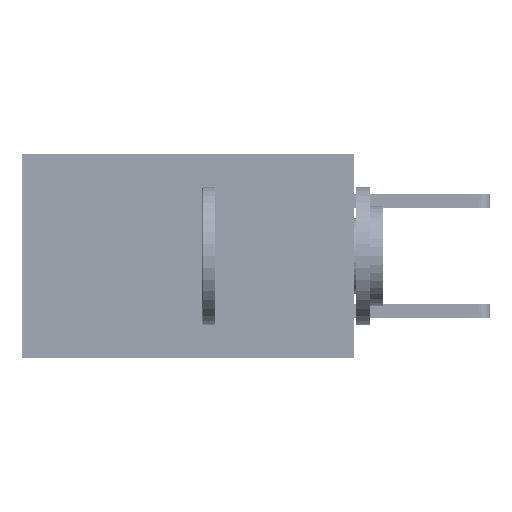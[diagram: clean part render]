
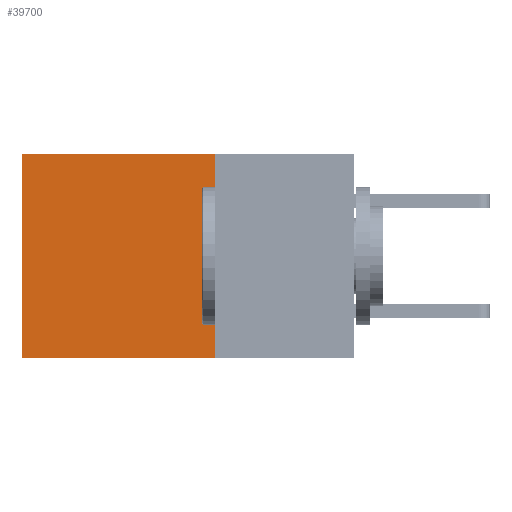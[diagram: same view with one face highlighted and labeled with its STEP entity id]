
A CAD part, left-side view. The second image highlights one B-rep face of the part: STEP entity #39700.
In plain terms, the highlighted planar face has unit normal (-1, 0, 0).
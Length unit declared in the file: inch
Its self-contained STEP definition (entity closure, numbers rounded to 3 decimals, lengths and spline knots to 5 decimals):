
#5642 = EDGE_LOOP ( 'NONE', ( #17971, #10658, #11846, #21129 ) ) ;
#6318 = CARTESIAN_POINT ( 'NONE',  ( 0.2875, 0.25, 0. ) ) ;
#7401 = CARTESIAN_POINT ( 'NONE',  ( 0.2875, 0.6, -0.37 ) ) ;
#7783 = FACE_OUTER_BOUND ( 'NONE', #5642, .T. ) ;
#10658 = ORIENTED_EDGE ( 'NONE', *, *, #20446, .F. ) ;
#11663 = VERTEX_POINT ( 'NONE', #6318 ) ;
#11846 = ORIENTED_EDGE ( 'NONE', *, *, #44434, .F. ) ;
#13267 = LINE ( 'NONE', #27646, #29288 ) ;
#13630 = VERTEX_POINT ( 'NONE', #45906 ) ;
#15787 = CARTESIAN_POINT ( 'NONE',  ( 0.2875, 0.25, 0. ) ) ;
#15796 = LINE ( 'NONE', #33018, #42205 ) ;
#16317 = VECTOR ( 'NONE', #34001, 39.37008 ) ;
#17438 = VERTEX_POINT ( 'NONE', #7401 ) ;
#17971 = ORIENTED_EDGE ( 'NONE', *, *, #22634, .T. ) ;
#20446 = EDGE_CURVE ( 'NONE', #41183, #17438, #13267, .T. ) ;
#21129 = ORIENTED_EDGE ( 'NONE', *, *, #32386, .T. ) ;
#22634 = EDGE_CURVE ( 'NONE', #13630, #17438, #15796, .T. ) ;
#23850 = DIRECTION ( 'NONE',  ( 0., 0., -1. ) ) ;
#24641 = AXIS2_PLACEMENT_3D ( 'NONE', #15787, #40311, #30155 ) ;
#27170 = LINE ( 'NONE', #27402, #16317 ) ;
#27402 = CARTESIAN_POINT ( 'NONE',  ( 0.2875, 0.25, 0. ) ) ;
#27646 = CARTESIAN_POINT ( 'NONE',  ( 0.2875, 0.25, -0.37 ) ) ;
#29288 = VECTOR ( 'NONE', #42021, 39.37008 ) ;
#30155 = DIRECTION ( 'NONE',  ( 0., 0., -1. ) ) ;
#30162 = DIRECTION ( 'NONE',  ( 0., 0., -1. ) ) ;
#32386 = EDGE_CURVE ( 'NONE', #11663, #13630, #27170, .T. ) ;
#33018 = CARTESIAN_POINT ( 'NONE',  ( 0.2875, 0.6, 0. ) ) ;
#33744 = CARTESIAN_POINT ( 'NONE',  ( 0.2875, 0.25, 0. ) ) ;
#33968 = LINE ( 'NONE', #33744, #34885 ) ;
#34001 = DIRECTION ( 'NONE',  ( 0., 1., 0. ) ) ;
#34172 = CARTESIAN_POINT ( 'NONE',  ( 0.2875, 0.25, -0.37 ) ) ;
#34885 = VECTOR ( 'NONE', #23850, 39.37008 ) ;
#39700 = ADVANCED_FACE ( 'NONE', ( #7783 ), #44325, .F. ) ;
#40311 = DIRECTION ( 'NONE',  ( 1., 0., 0. ) ) ;
#41183 = VERTEX_POINT ( 'NONE', #34172 ) ;
#42021 = DIRECTION ( 'NONE',  ( 0., 1., 0. ) ) ;
#42205 = VECTOR ( 'NONE', #30162, 39.37008 ) ;
#44325 = PLANE ( 'NONE',  #24641 ) ;
#44434 = EDGE_CURVE ( 'NONE', #11663, #41183, #33968, .T. ) ;
#45906 = CARTESIAN_POINT ( 'NONE',  ( 0.2875, 0.6, 0. ) ) ;
